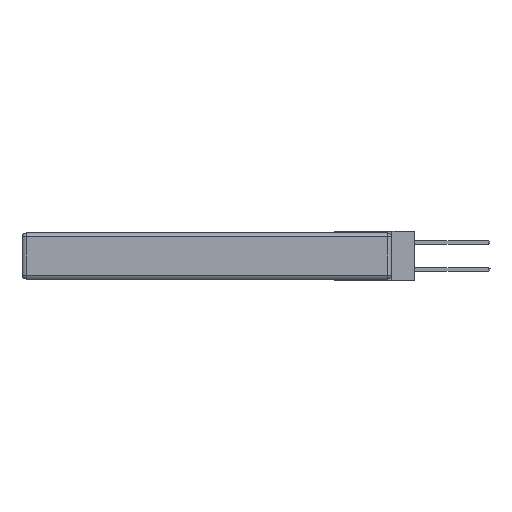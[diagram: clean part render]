
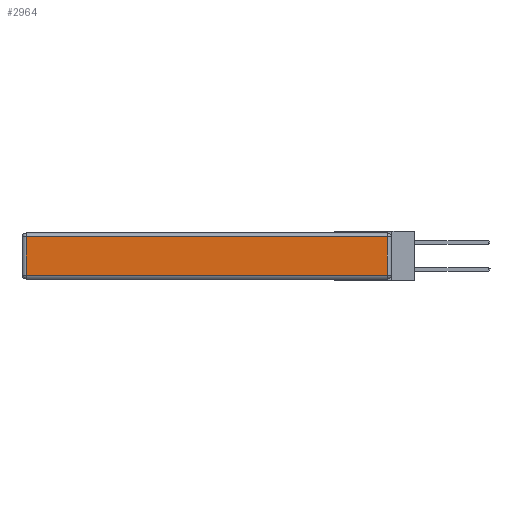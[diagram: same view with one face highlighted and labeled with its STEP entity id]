
A CAD part, left-side view. The second image highlights one B-rep face of the part: STEP entity #2964.
In plain terms, the highlighted planar face has unit normal (-1, 0, 0).
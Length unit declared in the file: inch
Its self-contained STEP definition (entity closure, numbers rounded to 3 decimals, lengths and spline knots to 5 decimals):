
#400 = FACE_OUTER_BOUND ( 'NONE', #15841, .T. ) ;
#644 = VERTEX_POINT ( 'NONE', #18891 ) ;
#1039 = VECTOR ( 'NONE', #14827, 39.37008 ) ;
#2964 = ADVANCED_FACE ( 'NONE', ( #400 ), #12313, .T. ) ;
#6626 = AXIS2_PLACEMENT_3D ( 'NONE', #15126, #34645, #20741 ) ;
#7415 = LINE ( 'NONE', #31366, #28811 ) ;
#7973 = EDGE_CURVE ( 'NONE', #33677, #9606, #23310, .T. ) ;
#9334 = LINE ( 'NONE', #26692, #22446 ) ;
#9606 = VERTEX_POINT ( 'NONE', #20397 ) ;
#11114 = CARTESIAN_POINT ( 'NONE',  ( 0., 2.72, -0.313 ) ) ;
#12072 = ORIENTED_EDGE ( 'NONE', *, *, #30142, .T. ) ;
#12148 = LINE ( 'NONE', #32683, #30954 ) ;
#12313 = PLANE ( 'NONE',  #6626 ) ;
#13996 = CARTESIAN_POINT ( 'NONE',  ( 0., 0., -0.313 ) ) ;
#14827 = DIRECTION ( 'NONE',  ( 0., -1., 0. ) ) ;
#15126 = CARTESIAN_POINT ( 'NONE',  ( 0., 0., -0.343 ) ) ;
#15485 = DIRECTION ( 'NONE',  ( 0., 0., 1. ) ) ;
#15841 = EDGE_LOOP ( 'NONE', ( #15869, #12072, #32371, #29351 ) ) ;
#15869 = ORIENTED_EDGE ( 'NONE', *, *, #7973, .T. ) ;
#17660 = EDGE_CURVE ( 'NONE', #644, #33677, #12148, .T. ) ;
#18891 = CARTESIAN_POINT ( 'NONE',  ( 0., 2.72, -0.03 ) ) ;
#20397 = CARTESIAN_POINT ( 'NONE',  ( 0., 0.03, -0.313 ) ) ;
#20741 = DIRECTION ( 'NONE',  ( 0., 0., 1. ) ) ;
#22446 = VECTOR ( 'NONE', #24249, 39.37008 ) ;
#23004 = VERTEX_POINT ( 'NONE', #29863 ) ;
#23310 = LINE ( 'NONE', #13996, #1039 ) ;
#24249 = DIRECTION ( 'NONE',  ( 0., 1., 0. ) ) ;
#25079 = DIRECTION ( 'NONE',  ( 0., 0., -1. ) ) ;
#26692 = CARTESIAN_POINT ( 'NONE',  ( 0., 2.75, -0.03 ) ) ;
#28811 = VECTOR ( 'NONE', #15485, 39.37008 ) ;
#29351 = ORIENTED_EDGE ( 'NONE', *, *, #17660, .T. ) ;
#29863 = CARTESIAN_POINT ( 'NONE',  ( 0., 0.03, -0.03 ) ) ;
#30142 = EDGE_CURVE ( 'NONE', #9606, #23004, #7415, .T. ) ;
#30954 = VECTOR ( 'NONE', #25079, 39.37008 ) ;
#31366 = CARTESIAN_POINT ( 'NONE',  ( 0., 0.03, -0.343 ) ) ;
#32371 = ORIENTED_EDGE ( 'NONE', *, *, #33824, .T. ) ;
#32683 = CARTESIAN_POINT ( 'NONE',  ( 0., 2.72, -0.343 ) ) ;
#33677 = VERTEX_POINT ( 'NONE', #11114 ) ;
#33824 = EDGE_CURVE ( 'NONE', #23004, #644, #9334, .T. ) ;
#34645 = DIRECTION ( 'NONE',  ( -1., 0., 0. ) ) ;
